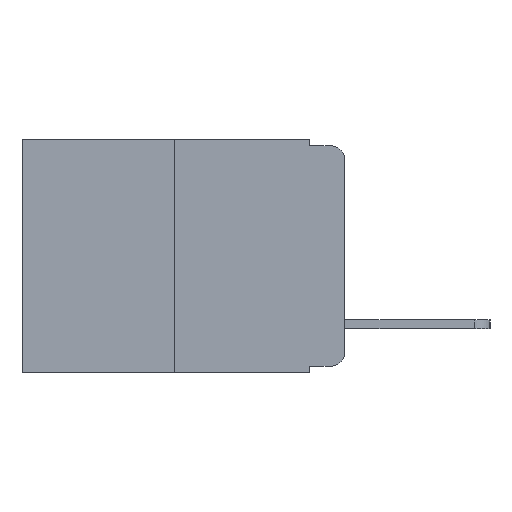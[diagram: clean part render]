
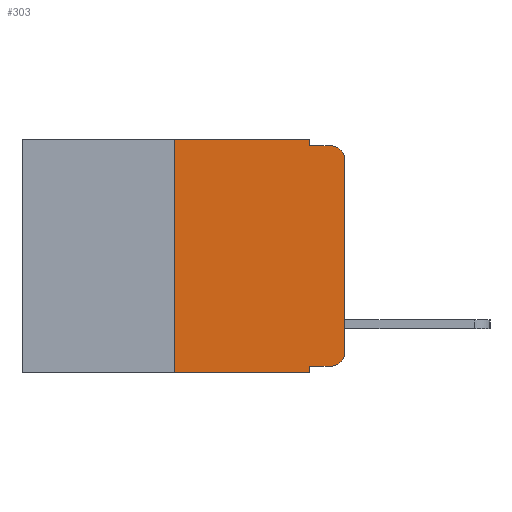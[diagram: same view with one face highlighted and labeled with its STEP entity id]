
A CAD part, left-side view. The second image highlights one B-rep face of the part: STEP entity #303.
In plain terms, the highlighted planar face has unit normal (-1, 0, 0).
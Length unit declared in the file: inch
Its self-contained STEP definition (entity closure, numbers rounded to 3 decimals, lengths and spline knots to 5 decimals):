
#171 = CARTESIAN_POINT ( 'NONE',  ( 0., 0.25, 0. ) ) ;
#303 = ADVANCED_FACE ( 'NONE', ( #13251 ), #15827, .F. ) ;
#459 = EDGE_CURVE ( 'NONE', #2635, #1464, #3506, .T. ) ;
#615 = DIRECTION ( 'NONE',  ( 0., 0., 1. ) ) ;
#1141 = ORIENTED_EDGE ( 'NONE', *, *, #9585, .F. ) ;
#1241 = CARTESIAN_POINT ( 'NONE',  ( 0., 0.051, -0.333 ) ) ;
#1309 = VERTEX_POINT ( 'NONE', #10931 ) ;
#1464 = VERTEX_POINT ( 'NONE', #9404 ) ;
#2038 = ORIENTED_EDGE ( 'NONE', *, *, #10807, .T. ) ;
#2111 = VERTEX_POINT ( 'NONE', #11714 ) ;
#2299 = AXIS2_PLACEMENT_3D ( 'NONE', #9137, #10881, #9183 ) ;
#2635 = VERTEX_POINT ( 'NONE', #171 ) ;
#2839 = EDGE_CURVE ( 'NONE', #1309, #2635, #9209, .T. ) ;
#2896 = CARTESIAN_POINT ( 'NONE',  ( 0., 0.051, -0.01 ) ) ;
#2995 = ORIENTED_EDGE ( 'NONE', *, *, #2839, .F. ) ;
#3241 = LINE ( 'NONE', #8319, #15155 ) ;
#3383 = CARTESIAN_POINT ( 'NONE',  ( 0., 0.051, -0.01 ) ) ;
#3467 = VERTEX_POINT ( 'NONE', #6533 ) ;
#3506 = LINE ( 'NONE', #10969, #6452 ) ;
#3579 = LINE ( 'NONE', #3383, #7249 ) ;
#3609 = CARTESIAN_POINT ( 'NONE',  ( 0., 0.02, -0.03 ) ) ;
#3656 = LINE ( 'NONE', #8815, #9740 ) ;
#3697 = ORIENTED_EDGE ( 'NONE', *, *, #6856, .T. ) ;
#3993 = ORIENTED_EDGE ( 'NONE', *, *, #7994, .T. ) ;
#4662 = DIRECTION ( 'NONE',  ( 0., -1., 0. ) ) ;
#4714 = AXIS2_PLACEMENT_3D ( 'NONE', #3609, #12040, #4892 ) ;
#4892 = DIRECTION ( 'NONE',  ( 0., 0., -1. ) ) ;
#5090 = ORIENTED_EDGE ( 'NONE', *, *, #459, .F. ) ;
#5228 = CARTESIAN_POINT ( 'NONE',  ( 0., 0.25, 0. ) ) ;
#5439 = EDGE_CURVE ( 'NONE', #12394, #5692, #12618, .T. ) ;
#5666 = VECTOR ( 'NONE', #8204, 39.37008 ) ;
#5692 = VERTEX_POINT ( 'NONE', #15271 ) ;
#5836 = EDGE_LOOP ( 'NONE', ( #3993, #13869, #7647, #9825, #5090, #2995, #2038, #1141, #3697, #6715 ) ) ;
#6082 = LINE ( 'NONE', #8349, #9612 ) ;
#6452 = VECTOR ( 'NONE', #10766, 39.37008 ) ;
#6459 = LINE ( 'NONE', #15270, #15418 ) ;
#6533 = CARTESIAN_POINT ( 'NONE',  ( 0., 0.02, -0.01 ) ) ;
#6643 = DIRECTION ( 'NONE',  ( -1., 0., 0. ) ) ;
#6715 = ORIENTED_EDGE ( 'NONE', *, *, #5439, .T. ) ;
#6856 = EDGE_CURVE ( 'NONE', #14279, #12394, #15841, .T. ) ;
#6950 = EDGE_CURVE ( 'NONE', #9096, #3467, #3579, .T. ) ;
#7249 = VECTOR ( 'NONE', #4662, 39.37008 ) ;
#7647 = ORIENTED_EDGE ( 'NONE', *, *, #6950, .F. ) ;
#7972 = EDGE_CURVE ( 'NONE', #1464, #9096, #6459, .T. ) ;
#7994 = EDGE_CURVE ( 'NONE', #5692, #9276, #6082, .T. ) ;
#8204 = DIRECTION ( 'NONE',  ( 0., 0., 1. ) ) ;
#8319 = CARTESIAN_POINT ( 'NONE',  ( 0., 0.473, -0.343 ) ) ;
#8349 = CARTESIAN_POINT ( 'NONE',  ( 0., 0., 0. ) ) ;
#8815 = CARTESIAN_POINT ( 'NONE',  ( 0., 0.051, 0. ) ) ;
#9096 = VERTEX_POINT ( 'NONE', #2896 ) ;
#9137 = CARTESIAN_POINT ( 'NONE',  ( 0., 0.473, 0. ) ) ;
#9183 = DIRECTION ( 'NONE',  ( 0., 0., -1. ) ) ;
#9209 = LINE ( 'NONE', #5228, #5666 ) ;
#9276 = VERTEX_POINT ( 'NONE', #10629 ) ;
#9404 = CARTESIAN_POINT ( 'NONE',  ( 0., 0.051, 0. ) ) ;
#9585 = EDGE_CURVE ( 'NONE', #14279, #2111, #3656, .T. ) ;
#9612 = VECTOR ( 'NONE', #615, 39.37008 ) ;
#9740 = VECTOR ( 'NONE', #14593, 39.37008 ) ;
#9825 = ORIENTED_EDGE ( 'NONE', *, *, #7972, .F. ) ;
#10032 = AXIS2_PLACEMENT_3D ( 'NONE', #13653, #6643, #14799 ) ;
#10617 = DIRECTION ( 'NONE',  ( 0., 0., -1. ) ) ;
#10629 = CARTESIAN_POINT ( 'NONE',  ( 0., 0., -0.03 ) ) ;
#10766 = DIRECTION ( 'NONE',  ( 0., -1., 0. ) ) ;
#10807 = EDGE_CURVE ( 'NONE', #1309, #2111, #3241, .T. ) ;
#10881 = DIRECTION ( 'NONE',  ( 1., 0., 0. ) ) ;
#10931 = CARTESIAN_POINT ( 'NONE',  ( 0., 0.25, -0.343 ) ) ;
#10969 = CARTESIAN_POINT ( 'NONE',  ( 0., 0.473, 0. ) ) ;
#11090 = CIRCLE ( 'NONE', #4714, 0.02 ) ;
#11677 = DIRECTION ( 'NONE',  ( 0., -1., 0. ) ) ;
#11714 = CARTESIAN_POINT ( 'NONE',  ( 0., 0.051, -0.343 ) ) ;
#11887 = DIRECTION ( 'NONE',  ( 0., -1., 0. ) ) ;
#12040 = DIRECTION ( 'NONE',  ( -1., 0., 0. ) ) ;
#12394 = VERTEX_POINT ( 'NONE', #14525 ) ;
#12618 = CIRCLE ( 'NONE', #10032, 0.02 ) ;
#12786 = VECTOR ( 'NONE', #11677, 39.37008 ) ;
#13251 = FACE_OUTER_BOUND ( 'NONE', #5836, .T. ) ;
#13653 = CARTESIAN_POINT ( 'NONE',  ( 0., 0.02, -0.313 ) ) ;
#13869 = ORIENTED_EDGE ( 'NONE', *, *, #14694, .T. ) ;
#14279 = VERTEX_POINT ( 'NONE', #1241 ) ;
#14525 = CARTESIAN_POINT ( 'NONE',  ( 0., 0.02, -0.333 ) ) ;
#14593 = DIRECTION ( 'NONE',  ( 0., 0., -1. ) ) ;
#14694 = EDGE_CURVE ( 'NONE', #9276, #3467, #11090, .T. ) ;
#14799 = DIRECTION ( 'NONE',  ( 0., 0., -1. ) ) ;
#15070 = CARTESIAN_POINT ( 'NONE',  ( 0., 0.051, -0.333 ) ) ;
#15155 = VECTOR ( 'NONE', #11887, 39.37008 ) ;
#15270 = CARTESIAN_POINT ( 'NONE',  ( 0., 0.051, 0. ) ) ;
#15271 = CARTESIAN_POINT ( 'NONE',  ( 0., 0., -0.313 ) ) ;
#15418 = VECTOR ( 'NONE', #10617, 39.37008 ) ;
#15827 = PLANE ( 'NONE',  #2299 ) ;
#15841 = LINE ( 'NONE', #15070, #12786 ) ;
